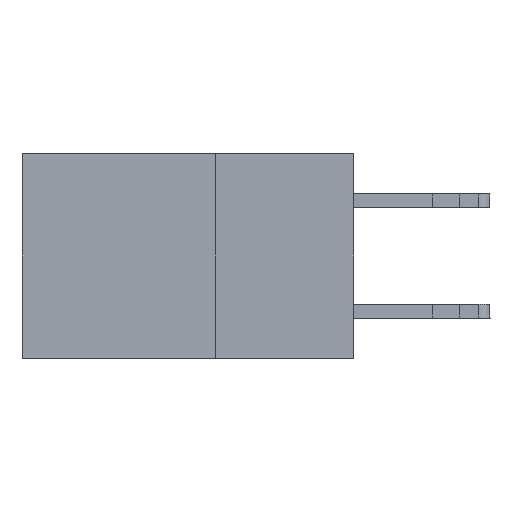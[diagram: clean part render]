
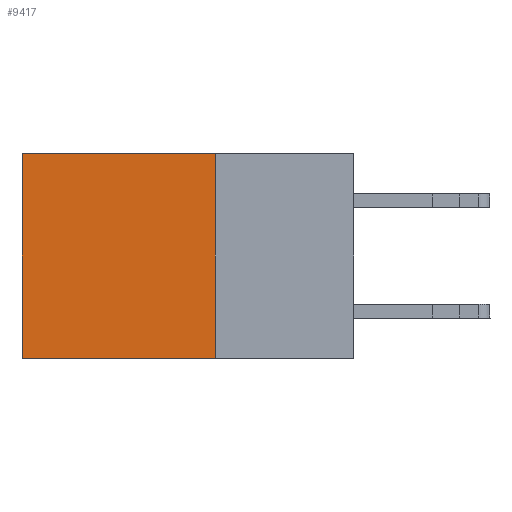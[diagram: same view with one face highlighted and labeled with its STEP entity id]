
A CAD part, left-side view. The second image highlights one B-rep face of the part: STEP entity #9417.
In plain terms, the highlighted planar face has unit normal (-1, 0, 0).
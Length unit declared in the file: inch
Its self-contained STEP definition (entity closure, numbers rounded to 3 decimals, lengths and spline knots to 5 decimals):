
#239 = DIRECTION ( 'NONE',  ( 0., 0., -1. ) ) ;
#589 = DIRECTION ( 'NONE',  ( 0., 0., -1. ) ) ;
#2406 = VECTOR ( 'NONE', #239, 39.37008 ) ;
#2772 = FACE_OUTER_BOUND ( 'NONE', #20896, .T. ) ;
#2858 = DIRECTION ( 'NONE',  ( 0., 1., 0. ) ) ;
#2894 = CARTESIAN_POINT ( 'NONE',  ( 0.2875, 0.25, 0. ) ) ;
#4117 = VECTOR ( 'NONE', #2858, 39.37008 ) ;
#4589 = VERTEX_POINT ( 'NONE', #20456 ) ;
#4887 = CARTESIAN_POINT ( 'NONE',  ( 0.2875, 0.6, -0.37 ) ) ;
#5469 = EDGE_CURVE ( 'NONE', #4589, #8139, #18574, .T. ) ;
#6059 = DIRECTION ( 'NONE',  ( 0., 0., -1. ) ) ;
#7323 = CARTESIAN_POINT ( 'NONE',  ( 0.2875, 0.25, -0.37 ) ) ;
#7492 = VERTEX_POINT ( 'NONE', #2894 ) ;
#7656 = CARTESIAN_POINT ( 'NONE',  ( 0.2875, 0.25, 0. ) ) ;
#8139 = VERTEX_POINT ( 'NONE', #4887 ) ;
#9226 = LINE ( 'NONE', #9539, #4117 ) ;
#9242 = PLANE ( 'NONE',  #15093 ) ;
#9316 = VECTOR ( 'NONE', #13923, 39.37008 ) ;
#9417 = ADVANCED_FACE ( 'NONE', ( #2772 ), #9242, .F. ) ;
#9539 = CARTESIAN_POINT ( 'NONE',  ( 0.2875, 0.25, 0. ) ) ;
#9634 = ORIENTED_EDGE ( 'NONE', *, *, #9838, .T. ) ;
#9838 = EDGE_CURVE ( 'NONE', #19975, #8139, #14498, .T. ) ;
#10942 = DIRECTION ( 'NONE',  ( 1., 0., 0. ) ) ;
#11299 = VECTOR ( 'NONE', #589, 39.37008 ) ;
#11496 = CARTESIAN_POINT ( 'NONE',  ( 0.2875, 0.6, 0. ) ) ;
#12590 = ORIENTED_EDGE ( 'NONE', *, *, #15606, .T. ) ;
#13923 = DIRECTION ( 'NONE',  ( 0., 1., 0. ) ) ;
#14498 = LINE ( 'NONE', #11496, #2406 ) ;
#14772 = LINE ( 'NONE', #16253, #11299 ) ;
#15093 = AXIS2_PLACEMENT_3D ( 'NONE', #7656, #10942, #6059 ) ;
#15606 = EDGE_CURVE ( 'NONE', #7492, #19975, #9226, .T. ) ;
#16253 = CARTESIAN_POINT ( 'NONE',  ( 0.2875, 0.25, 0. ) ) ;
#16363 = CARTESIAN_POINT ( 'NONE',  ( 0.2875, 0.6, 0. ) ) ;
#16988 = ORIENTED_EDGE ( 'NONE', *, *, #5469, .F. ) ;
#18574 = LINE ( 'NONE', #7323, #9316 ) ;
#18591 = EDGE_CURVE ( 'NONE', #7492, #4589, #14772, .T. ) ;
#19356 = ORIENTED_EDGE ( 'NONE', *, *, #18591, .F. ) ;
#19975 = VERTEX_POINT ( 'NONE', #16363 ) ;
#20456 = CARTESIAN_POINT ( 'NONE',  ( 0.2875, 0.25, -0.37 ) ) ;
#20896 = EDGE_LOOP ( 'NONE', ( #9634, #16988, #19356, #12590 ) ) ;
